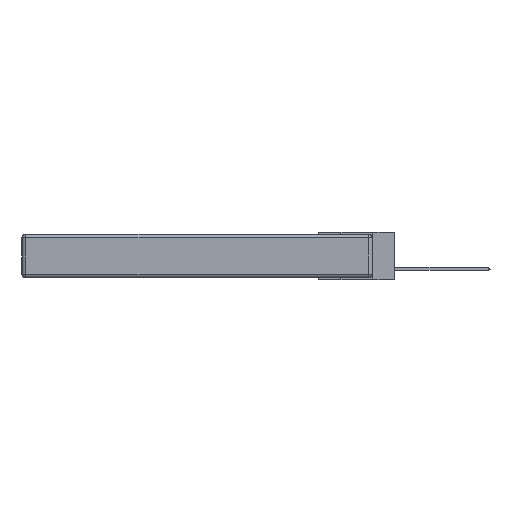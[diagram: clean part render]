
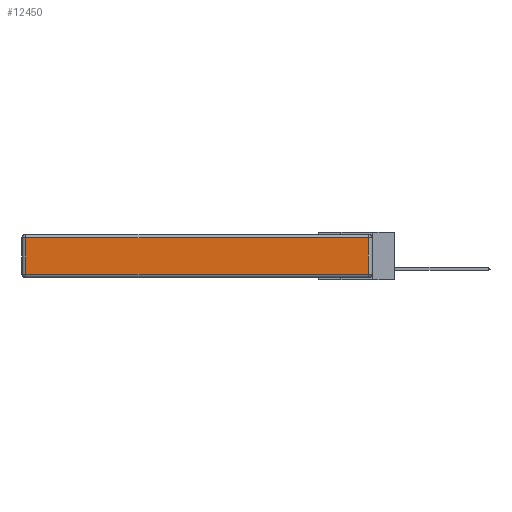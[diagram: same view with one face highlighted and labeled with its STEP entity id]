
A CAD part, left-side view. The second image highlights one B-rep face of the part: STEP entity #12450.
In plain terms, the highlighted planar face has unit normal (-1, 0, 0).
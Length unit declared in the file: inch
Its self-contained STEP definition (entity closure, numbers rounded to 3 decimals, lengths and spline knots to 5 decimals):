
#150 = ORIENTED_EDGE ( 'NONE', *, *, #12841, .T. ) ;
#1695 = EDGE_CURVE ( 'NONE', #18198, #17239, #19496, .T. ) ;
#2154 = DIRECTION ( 'NONE',  ( 0., 0., 1. ) ) ;
#3100 = EDGE_CURVE ( 'NONE', #17239, #8969, #6601, .T. ) ;
#4959 = LINE ( 'NONE', #17992, #20881 ) ;
#6601 = LINE ( 'NONE', #19979, #13737 ) ;
#6840 = CARTESIAN_POINT ( 'NONE',  ( 0., 2.72, -0.313 ) ) ;
#7634 = CARTESIAN_POINT ( 'NONE',  ( 0., 0.03, -0.03 ) ) ;
#8031 = EDGE_CURVE ( 'NONE', #8465, #18198, #4959, .T. ) ;
#8133 = DIRECTION ( 'NONE',  ( 0., 0., -1. ) ) ;
#8190 = DIRECTION ( 'NONE',  ( 0., -1., 0. ) ) ;
#8465 = VERTEX_POINT ( 'NONE', #6840 ) ;
#8934 = CARTESIAN_POINT ( 'NONE',  ( 0., 2.72, -0.03 ) ) ;
#8969 = VERTEX_POINT ( 'NONE', #8934 ) ;
#10233 = DIRECTION ( 'NONE',  ( -1., 0., 0. ) ) ;
#10799 = CARTESIAN_POINT ( 'NONE',  ( 0., 0.03, -0.313 ) ) ;
#10957 = ORIENTED_EDGE ( 'NONE', *, *, #3100, .T. ) ;
#11289 = CARTESIAN_POINT ( 'NONE',  ( 0., 2.72, -0.343 ) ) ;
#12450 = ADVANCED_FACE ( 'NONE', ( #20416 ), #18593, .T. ) ;
#12841 = EDGE_CURVE ( 'NONE', #8969, #8465, #20925, .T. ) ;
#13737 = VECTOR ( 'NONE', #16632, 39.37008 ) ;
#14522 = AXIS2_PLACEMENT_3D ( 'NONE', #16712, #10233, #2154 ) ;
#14820 = VECTOR ( 'NONE', #20048, 39.37008 ) ;
#15846 = ORIENTED_EDGE ( 'NONE', *, *, #1695, .T. ) ;
#16632 = DIRECTION ( 'NONE',  ( 0., 1., 0. ) ) ;
#16712 = CARTESIAN_POINT ( 'NONE',  ( 0., 0., -0.343 ) ) ;
#17239 = VERTEX_POINT ( 'NONE', #7634 ) ;
#17567 = VECTOR ( 'NONE', #8133, 39.37008 ) ;
#17992 = CARTESIAN_POINT ( 'NONE',  ( 0., 0., -0.313 ) ) ;
#18065 = EDGE_LOOP ( 'NONE', ( #19981, #15846, #10957, #150 ) ) ;
#18198 = VERTEX_POINT ( 'NONE', #10799 ) ;
#18539 = CARTESIAN_POINT ( 'NONE',  ( 0., 0.03, -0.343 ) ) ;
#18593 = PLANE ( 'NONE',  #14522 ) ;
#19496 = LINE ( 'NONE', #18539, #14820 ) ;
#19979 = CARTESIAN_POINT ( 'NONE',  ( 0., 2.75, -0.03 ) ) ;
#19981 = ORIENTED_EDGE ( 'NONE', *, *, #8031, .T. ) ;
#20048 = DIRECTION ( 'NONE',  ( 0., 0., 1. ) ) ;
#20416 = FACE_OUTER_BOUND ( 'NONE', #18065, .T. ) ;
#20881 = VECTOR ( 'NONE', #8190, 39.37008 ) ;
#20925 = LINE ( 'NONE', #11289, #17567 ) ;
